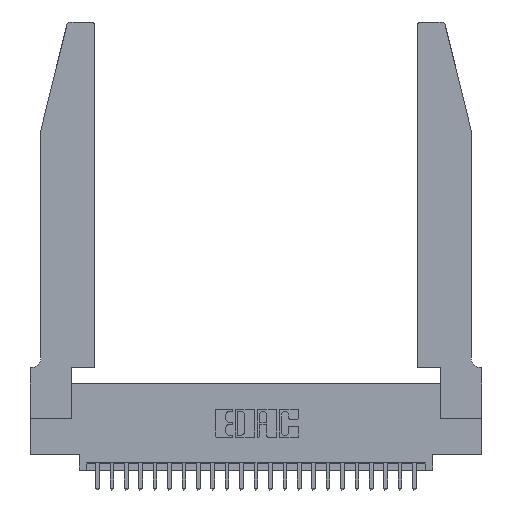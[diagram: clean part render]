
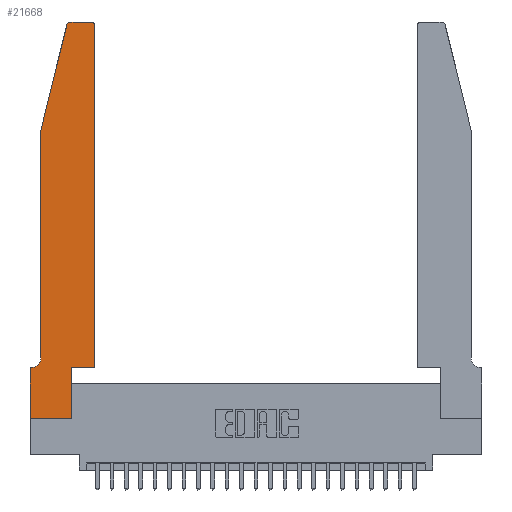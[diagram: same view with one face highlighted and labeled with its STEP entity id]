
A CAD part, top view. The second image highlights one B-rep face of the part: STEP entity #21668.
In plain terms, the highlighted planar face has unit normal (0, 0, 1).
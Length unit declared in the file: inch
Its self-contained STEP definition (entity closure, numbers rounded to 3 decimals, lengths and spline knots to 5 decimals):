
#141 = ORIENTED_EDGE ( 'NONE', *, *, #24102, .T. ) ;
#152 = ORIENTED_EDGE ( 'NONE', *, *, #5260, .T. ) ;
#220 = ORIENTED_EDGE ( 'NONE', *, *, #22378, .T. ) ;
#306 = EDGE_CURVE ( 'NONE', #3655, #8819, #18746, .T. ) ;
#334 = VERTEX_POINT ( 'NONE', #3244 ) ;
#547 = LINE ( 'NONE', #20590, #24063 ) ;
#843 = DIRECTION ( 'NONE',  ( -1., 0., 0. ) ) ;
#1315 = EDGE_CURVE ( 'NONE', #7208, #3655, #15654, .T. ) ;
#1376 = VECTOR ( 'NONE', #21316, 39.37008 ) ;
#1784 = CIRCLE ( 'NONE', #2395, 0.03 ) ;
#2151 = ORIENTED_EDGE ( 'NONE', *, *, #22334, .T. ) ;
#2367 = ORIENTED_EDGE ( 'NONE', *, *, #3751, .T. ) ;
#2395 = AXIS2_PLACEMENT_3D ( 'NONE', #15160, #3224, #17123 ) ;
#3078 = CARTESIAN_POINT ( 'NONE',  ( 0.4205, 2.72, 0.37 ) ) ;
#3224 = DIRECTION ( 'NONE',  ( 0., 0., 1. ) ) ;
#3244 = CARTESIAN_POINT ( 'NONE',  ( 0.2865, 0.35, 0.37 ) ) ;
#3655 = VERTEX_POINT ( 'NONE', #5359 ) ;
#3751 = EDGE_CURVE ( 'NONE', #17714, #6212, #17289, .T. ) ;
#4169 = CARTESIAN_POINT ( 'NONE',  ( 0., 0.35, 0.37 ) ) ;
#4447 = LINE ( 'NONE', #12128, #15040 ) ;
#4553 = VERTEX_POINT ( 'NONE', #24248 ) ;
#5019 = DIRECTION ( 'NONE',  ( 1., 0., 0. ) ) ;
#5038 = AXIS2_PLACEMENT_3D ( 'NONE', #24474, #12923, #843 ) ;
#5099 = VECTOR ( 'NONE', #13849, 39.37008 ) ;
#5114 = DIRECTION ( 'NONE',  ( 1., 0., 0. ) ) ;
#5260 = EDGE_CURVE ( 'NONE', #17886, #11266, #18166, .T. ) ;
#5359 = CARTESIAN_POINT ( 'NONE',  ( 0., 0., 0.37 ) ) ;
#6212 = VERTEX_POINT ( 'NONE', #6407 ) ;
#6214 = DIRECTION ( 'NONE',  ( 0., 0., 1. ) ) ;
#6407 = CARTESIAN_POINT ( 'NONE',  ( 0.4505, 2.72, 0.37 ) ) ;
#6618 = CARTESIAN_POINT ( 'NONE',  ( 0., 0., 0.37 ) ) ;
#6798 = DIRECTION ( 'NONE',  ( -0.239, -0.971, 0. ) ) ;
#6814 = EDGE_CURVE ( 'NONE', #11266, #24921, #4447, .T. ) ;
#6902 = DIRECTION ( 'NONE',  ( 0., 1., 0. ) ) ;
#7208 = VERTEX_POINT ( 'NONE', #11187 ) ;
#7267 = LINE ( 'NONE', #15855, #12570 ) ;
#7477 = CARTESIAN_POINT ( 'NONE',  ( 0.25487, 2.72718, 0.37 ) ) ;
#8551 = CIRCLE ( 'NONE', #10628, 0.03 ) ;
#8819 = VERTEX_POINT ( 'NONE', #22119 ) ;
#8912 = VERTEX_POINT ( 'NONE', #14696 ) ;
#9146 = FACE_OUTER_BOUND ( 'NONE', #11017, .T. ) ;
#9174 = VECTOR ( 'NONE', #11525, 39.37008 ) ;
#9511 = LINE ( 'NONE', #17522, #14758 ) ;
#9665 = CARTESIAN_POINT ( 'NONE',  ( 0.4505, 0.35, 0.37 ) ) ;
#9687 = EDGE_CURVE ( 'NONE', #23577, #17886, #1784, .T. ) ;
#9937 = DIRECTION ( 'NONE',  ( -1., 0., 0. ) ) ;
#10628 = AXIS2_PLACEMENT_3D ( 'NONE', #3078, #16990, #5114 ) ;
#10633 = ORIENTED_EDGE ( 'NONE', *, *, #20615, .T. ) ;
#10829 = ORIENTED_EDGE ( 'NONE', *, *, #14335, .T. ) ;
#11013 = ORIENTED_EDGE ( 'NONE', *, *, #25318, .T. ) ;
#11017 = EDGE_LOOP ( 'NONE', ( #10829, #18697, #152, #23509, #10633, #11013, #17995, #17553, #2151, #141, #2367, #220 ) ) ;
#11187 = CARTESIAN_POINT ( 'NONE',  ( 0., 0.35, 0.37 ) ) ;
#11266 = VERTEX_POINT ( 'NONE', #22327 ) ;
#11525 = DIRECTION ( 'NONE',  ( -1., 0., 0. ) ) ;
#12128 = CARTESIAN_POINT ( 'NONE',  ( 0.0755, 2., 0.37 ) ) ;
#12570 = VECTOR ( 'NONE', #9937, 39.37008 ) ;
#12757 = CARTESIAN_POINT ( 'NONE',  ( 0.0755, 2., 0.37 ) ) ;
#12923 = DIRECTION ( 'NONE',  ( 0., 0., -1. ) ) ;
#12961 = AXIS2_PLACEMENT_3D ( 'NONE', #4169, #6214, #19940 ) ;
#13849 = DIRECTION ( 'NONE',  ( 0., -1., 0. ) ) ;
#14335 = EDGE_CURVE ( 'NONE', #8912, #23577, #24688, .T. ) ;
#14696 = CARTESIAN_POINT ( 'NONE',  ( 0.4205, 2.75, 0.37 ) ) ;
#14758 = VECTOR ( 'NONE', #23312, 39.37008 ) ;
#14911 = CARTESIAN_POINT ( 'NONE',  ( 0.4505, 0.35, 0.37 ) ) ;
#15040 = VECTOR ( 'NONE', #21704, 39.37008 ) ;
#15160 = CARTESIAN_POINT ( 'NONE',  ( 0.284, 2.72, 0.37 ) ) ;
#15654 = LINE ( 'NONE', #16884, #5099 ) ;
#15855 = CARTESIAN_POINT ( 'NONE',  ( 0.0755, 0.35, 0.37 ) ) ;
#16083 = PLANE ( 'NONE',  #12961 ) ;
#16884 = CARTESIAN_POINT ( 'NONE',  ( 0., 0., 0.37 ) ) ;
#16959 = VECTOR ( 'NONE', #6798, 39.37008 ) ;
#16990 = DIRECTION ( 'NONE',  ( 0., 0., 1. ) ) ;
#17123 = DIRECTION ( 'NONE',  ( 1., 0., 0. ) ) ;
#17289 = LINE ( 'NONE', #9665, #1376 ) ;
#17522 = CARTESIAN_POINT ( 'NONE',  ( 0.4505, 0.35, 0.37 ) ) ;
#17537 = VECTOR ( 'NONE', #5019, 39.37008 ) ;
#17553 = ORIENTED_EDGE ( 'NONE', *, *, #306, .T. ) ;
#17714 = VERTEX_POINT ( 'NONE', #14911 ) ;
#17886 = VERTEX_POINT ( 'NONE', #7477 ) ;
#17995 = ORIENTED_EDGE ( 'NONE', *, *, #1315, .T. ) ;
#18166 = LINE ( 'NONE', #12757, #16959 ) ;
#18669 = CARTESIAN_POINT ( 'NONE',  ( 0.0755, 0.42, 0.37 ) ) ;
#18697 = ORIENTED_EDGE ( 'NONE', *, *, #9687, .T. ) ;
#18746 = LINE ( 'NONE', #6618, #17537 ) ;
#19940 = DIRECTION ( 'NONE',  ( 1., 0., 0. ) ) ;
#20590 = CARTESIAN_POINT ( 'NONE',  ( 0.2865, 0.35, 0.37 ) ) ;
#20615 = EDGE_CURVE ( 'NONE', #24921, #4553, #25309, .T. ) ;
#21060 = CARTESIAN_POINT ( 'NONE',  ( 0.2605, 2.75, 0.37 ) ) ;
#21316 = DIRECTION ( 'NONE',  ( 0., 1., 0. ) ) ;
#21668 = ADVANCED_FACE ( 'NONE', ( #9146 ), #16083, .T. ) ;
#21704 = DIRECTION ( 'NONE',  ( 0., -1., 0. ) ) ;
#22119 = CARTESIAN_POINT ( 'NONE',  ( 0.2865, 0., 0.37 ) ) ;
#22327 = CARTESIAN_POINT ( 'NONE',  ( 0.0755, 2., 0.37 ) ) ;
#22334 = EDGE_CURVE ( 'NONE', #8819, #334, #547, .T. ) ;
#22378 = EDGE_CURVE ( 'NONE', #6212, #8912, #8551, .T. ) ;
#23312 = DIRECTION ( 'NONE',  ( 1., 0., 0. ) ) ;
#23509 = ORIENTED_EDGE ( 'NONE', *, *, #6814, .T. ) ;
#23577 = VERTEX_POINT ( 'NONE', #23763 ) ;
#23763 = CARTESIAN_POINT ( 'NONE',  ( 0.284, 2.75, 0.37 ) ) ;
#24063 = VECTOR ( 'NONE', #6902, 39.37008 ) ;
#24102 = EDGE_CURVE ( 'NONE', #334, #17714, #9511, .T. ) ;
#24248 = CARTESIAN_POINT ( 'NONE',  ( 0.0055, 0.35, 0.37 ) ) ;
#24474 = CARTESIAN_POINT ( 'NONE',  ( 0.0055, 0.42, 0.37 ) ) ;
#24688 = LINE ( 'NONE', #21060, #9174 ) ;
#24921 = VERTEX_POINT ( 'NONE', #18669 ) ;
#25309 = CIRCLE ( 'NONE', #5038, 0.07 ) ;
#25318 = EDGE_CURVE ( 'NONE', #4553, #7208, #7267, .T. ) ;
